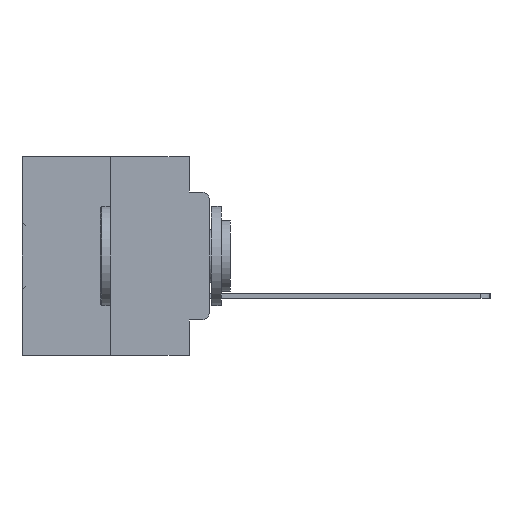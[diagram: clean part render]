
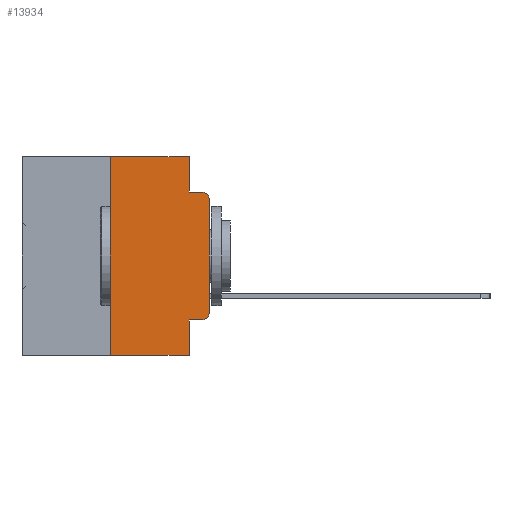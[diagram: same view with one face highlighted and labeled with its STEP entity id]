
A CAD part, left-side view. The second image highlights one B-rep face of the part: STEP entity #13934.
In plain terms, the highlighted planar face has unit normal (-1, 0, 0).
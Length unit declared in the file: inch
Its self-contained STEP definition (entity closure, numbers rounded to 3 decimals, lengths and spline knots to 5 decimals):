
#726 = LINE ( 'NONE', #27209, #8315 ) ;
#834 = CARTESIAN_POINT ( 'NONE',  ( 0., 0.051, -0.4115 ) ) ;
#1047 = CARTESIAN_POINT ( 'NONE',  ( 0., 0.051, -0.0885 ) ) ;
#1478 = VERTEX_POINT ( 'NONE', #28516 ) ;
#1549 = CARTESIAN_POINT ( 'NONE',  ( 0., 0.02, -0.0885 ) ) ;
#2212 = CARTESIAN_POINT ( 'NONE',  ( 0., 0.473, 0. ) ) ;
#3719 = DIRECTION ( 'NONE',  ( 0., -1., 0. ) ) ;
#4465 = CIRCLE ( 'NONE', #31162, 0.02 ) ;
#4917 = VECTOR ( 'NONE', #14179, 39.37008 ) ;
#5071 = DIRECTION ( 'NONE',  ( 0., -1., 0. ) ) ;
#5610 = CARTESIAN_POINT ( 'NONE',  ( 0., 0.473, 0. ) ) ;
#5726 = LINE ( 'NONE', #13244, #34219 ) ;
#6271 = VECTOR ( 'NONE', #5071, 39.37008 ) ;
#6498 = CARTESIAN_POINT ( 'NONE',  ( 0., 0.25, -0.5 ) ) ;
#6556 = AXIS2_PLACEMENT_3D ( 'NONE', #5610, #25597, #8481 ) ;
#7498 = VERTEX_POINT ( 'NONE', #29594 ) ;
#7886 = VERTEX_POINT ( 'NONE', #31419 ) ;
#7938 = AXIS2_PLACEMENT_3D ( 'NONE', #28484, #11459, #31309 ) ;
#8315 = VECTOR ( 'NONE', #24348, 39.37008 ) ;
#8436 = VECTOR ( 'NONE', #21087, 39.37008 ) ;
#8481 = DIRECTION ( 'NONE',  ( 0., 0., -1. ) ) ;
#8809 = VERTEX_POINT ( 'NONE', #21238 ) ;
#10435 = DIRECTION ( 'NONE',  ( -1., 0., 0. ) ) ;
#10785 = LINE ( 'NONE', #18062, #32509 ) ;
#11213 = EDGE_CURVE ( 'NONE', #26446, #28036, #15226, .T. ) ;
#11459 = DIRECTION ( 'NONE',  ( -1., 0., 0. ) ) ;
#12584 = LINE ( 'NONE', #14066, #4917 ) ;
#13242 = ORIENTED_EDGE ( 'NONE', *, *, #30249, .T. ) ;
#13244 = CARTESIAN_POINT ( 'NONE',  ( 0., 0.25, 0. ) ) ;
#13496 = ORIENTED_EDGE ( 'NONE', *, *, #20792, .T. ) ;
#13704 = ORIENTED_EDGE ( 'NONE', *, *, #11213, .F. ) ;
#13934 = ADVANCED_FACE ( 'NONE', ( #20789 ), #31134, .F. ) ;
#14019 = ORIENTED_EDGE ( 'NONE', *, *, #34718, .F. ) ;
#14066 = CARTESIAN_POINT ( 'NONE',  ( 0., 0., 0. ) ) ;
#14179 = DIRECTION ( 'NONE',  ( 0., 0., 1. ) ) ;
#14211 = ORIENTED_EDGE ( 'NONE', *, *, #29981, .F. ) ;
#14254 = ORIENTED_EDGE ( 'NONE', *, *, #22186, .F. ) ;
#14587 = EDGE_CURVE ( 'NONE', #7886, #19704, #726, .T. ) ;
#14665 = ORIENTED_EDGE ( 'NONE', *, *, #24604, .T. ) ;
#14784 = CARTESIAN_POINT ( 'NONE',  ( 0., 0.051, 0. ) ) ;
#14823 = ORIENTED_EDGE ( 'NONE', *, *, #14587, .F. ) ;
#15013 = CARTESIAN_POINT ( 'NONE',  ( 0., 0.051, -0.5 ) ) ;
#15204 = ORIENTED_EDGE ( 'NONE', *, *, #26686, .T. ) ;
#15226 = LINE ( 'NONE', #1047, #8436 ) ;
#15284 = ORIENTED_EDGE ( 'NONE', *, *, #24784, .T. ) ;
#15863 = LINE ( 'NONE', #14784, #34440 ) ;
#16739 = CARTESIAN_POINT ( 'NONE',  ( 0., 0., -0.1085 ) ) ;
#17958 = CIRCLE ( 'NONE', #7938, 0.02 ) ;
#18062 = CARTESIAN_POINT ( 'NONE',  ( 0., 0.473, -0.5 ) ) ;
#18954 = DIRECTION ( 'NONE',  ( 0., 0., 1. ) ) ;
#19704 = VERTEX_POINT ( 'NONE', #15013 ) ;
#20094 = VERTEX_POINT ( 'NONE', #16739 ) ;
#20789 = FACE_OUTER_BOUND ( 'NONE', #30715, .T. ) ;
#20792 = EDGE_CURVE ( 'NONE', #20094, #28036, #17958, .T. ) ;
#21087 = DIRECTION ( 'NONE',  ( 0., -1., 0. ) ) ;
#21238 = CARTESIAN_POINT ( 'NONE',  ( 0., 0.02, -0.4115 ) ) ;
#22186 = EDGE_CURVE ( 'NONE', #33649, #7498, #5726, .T. ) ;
#23317 = VECTOR ( 'NONE', #3719, 39.37008 ) ;
#24183 = LINE ( 'NONE', #834, #23317 ) ;
#24348 = DIRECTION ( 'NONE',  ( 0., 0., -1. ) ) ;
#24604 = EDGE_CURVE ( 'NONE', #33649, #19704, #10785, .T. ) ;
#24784 = EDGE_CURVE ( 'NONE', #8809, #25298, #4465, .T. ) ;
#24822 = CARTESIAN_POINT ( 'NONE',  ( 0., 0.051, -0.0885 ) ) ;
#25298 = VERTEX_POINT ( 'NONE', #26928 ) ;
#25597 = DIRECTION ( 'NONE',  ( 1., 0., 0. ) ) ;
#26446 = VERTEX_POINT ( 'NONE', #24822 ) ;
#26686 = EDGE_CURVE ( 'NONE', #7886, #8809, #24183, .T. ) ;
#26928 = CARTESIAN_POINT ( 'NONE',  ( 0., 0., -0.3915 ) ) ;
#27209 = CARTESIAN_POINT ( 'NONE',  ( 0., 0.051, 0. ) ) ;
#27466 = CARTESIAN_POINT ( 'NONE',  ( 0., 0.02, -0.3915 ) ) ;
#28036 = VERTEX_POINT ( 'NONE', #1549 ) ;
#28484 = CARTESIAN_POINT ( 'NONE',  ( 0., 0.02, -0.1085 ) ) ;
#28516 = CARTESIAN_POINT ( 'NONE',  ( 0., 0.051, 0. ) ) ;
#29017 = LINE ( 'NONE', #2212, #6271 ) ;
#29594 = CARTESIAN_POINT ( 'NONE',  ( 0., 0.25, 0. ) ) ;
#29981 = EDGE_CURVE ( 'NONE', #7498, #1478, #29017, .T. ) ;
#30249 = EDGE_CURVE ( 'NONE', #25298, #20094, #12584, .T. ) ;
#30295 = DIRECTION ( 'NONE',  ( 0., 0., -1. ) ) ;
#30715 = EDGE_LOOP ( 'NONE', ( #13242, #13496, #13704, #14019, #14211, #14254, #14665, #14823, #15204, #15284 ) ) ;
#31134 = PLANE ( 'NONE',  #6556 ) ;
#31162 = AXIS2_PLACEMENT_3D ( 'NONE', #27466, #10435, #30295 ) ;
#31309 = DIRECTION ( 'NONE',  ( 0., 0., -1. ) ) ;
#31419 = CARTESIAN_POINT ( 'NONE',  ( 0., 0.051, -0.4115 ) ) ;
#32509 = VECTOR ( 'NONE', #34964, 39.37008 ) ;
#33649 = VERTEX_POINT ( 'NONE', #6498 ) ;
#34219 = VECTOR ( 'NONE', #18954, 39.37008 ) ;
#34440 = VECTOR ( 'NONE', #34542, 39.37008 ) ;
#34542 = DIRECTION ( 'NONE',  ( 0., 0., -1. ) ) ;
#34718 = EDGE_CURVE ( 'NONE', #1478, #26446, #15863, .T. ) ;
#34964 = DIRECTION ( 'NONE',  ( 0., -1., 0. ) ) ;
